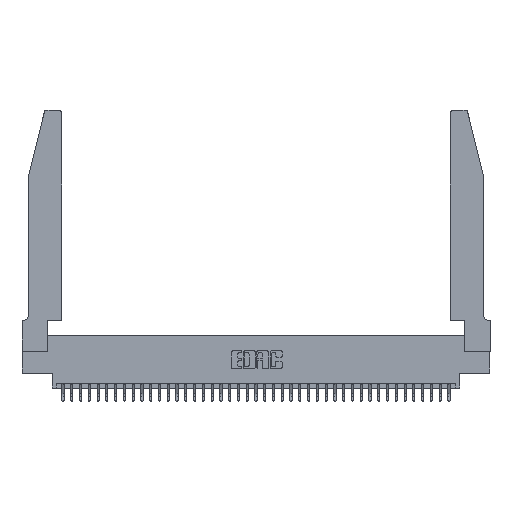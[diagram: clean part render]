
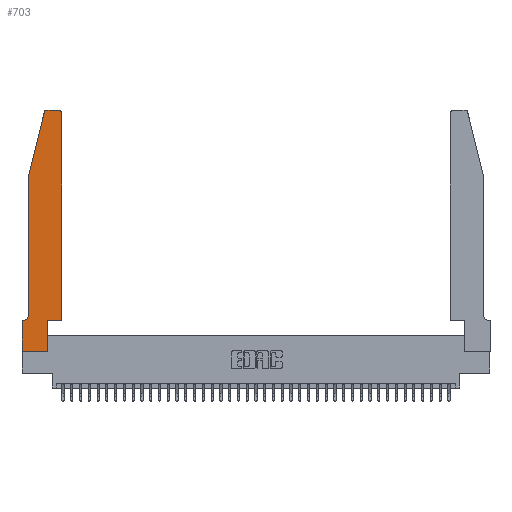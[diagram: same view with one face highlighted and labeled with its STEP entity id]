
A CAD part, top view. The second image highlights one B-rep face of the part: STEP entity #703.
In plain terms, the highlighted planar face has unit normal (0, 0, 1).
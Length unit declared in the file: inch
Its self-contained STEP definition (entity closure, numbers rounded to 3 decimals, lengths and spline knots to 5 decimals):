
#439 = LINE ( 'NONE', #4585, #27125 ) ;
#703 = ADVANCED_FACE ( 'NONE', ( #33845 ), #27674, .T. ) ;
#1113 = CARTESIAN_POINT ( 'NONE',  ( 0.2865, 0.35, 0.37 ) ) ;
#1779 = VECTOR ( 'NONE', #30031, 39.37008 ) ;
#1824 = AXIS2_PLACEMENT_3D ( 'NONE', #19420, #34696, #36988 ) ;
#2043 = CARTESIAN_POINT ( 'NONE',  ( 0., 0., 0.37 ) ) ;
#2507 = VERTEX_POINT ( 'NONE', #12022 ) ;
#2539 = VECTOR ( 'NONE', #35482, 39.37008 ) ;
#2873 = DIRECTION ( 'NONE',  ( -1., 0., 0. ) ) ;
#3063 = CARTESIAN_POINT ( 'NONE',  ( 0., 0., 0.37 ) ) ;
#3504 = VECTOR ( 'NONE', #10928, 39.37008 ) ;
#3772 = CARTESIAN_POINT ( 'NONE',  ( 0.0755, 0.35, 0.37 ) ) ;
#3827 = VERTEX_POINT ( 'NONE', #1113 ) ;
#4221 = CARTESIAN_POINT ( 'NONE',  ( 0.2865, 0., 0.37 ) ) ;
#4585 = CARTESIAN_POINT ( 'NONE',  ( 0.2605, 2.75, 0.37 ) ) ;
#4598 = EDGE_CURVE ( 'NONE', #10620, #25498, #7952, .T. ) ;
#5630 = LINE ( 'NONE', #7406, #1779 ) ;
#5864 = LINE ( 'NONE', #13849, #2539 ) ;
#6612 = EDGE_CURVE ( 'NONE', #27675, #13620, #20868, .T. ) ;
#7406 = CARTESIAN_POINT ( 'NONE',  ( 0.2865, 0.35, 0.37 ) ) ;
#7463 = EDGE_CURVE ( 'NONE', #13620, #33667, #439, .T. ) ;
#7952 = LINE ( 'NONE', #3772, #31646 ) ;
#8030 = ORIENTED_EDGE ( 'NONE', *, *, #7463, .T. ) ;
#8069 = LINE ( 'NONE', #9423, #23588 ) ;
#8191 = ORIENTED_EDGE ( 'NONE', *, *, #35374, .T. ) ;
#8224 = DIRECTION ( 'NONE',  ( 1., 0., 0. ) ) ;
#8551 = CIRCLE ( 'NONE', #23037, 0.07 ) ;
#8577 = ORIENTED_EDGE ( 'NONE', *, *, #36897, .T. ) ;
#8614 = DIRECTION ( 'NONE',  ( -1., 0., 0. ) ) ;
#8809 = CIRCLE ( 'NONE', #15777, 0.03 ) ;
#8848 = CARTESIAN_POINT ( 'NONE',  ( 0., 0.35, 0.37 ) ) ;
#9047 = ORIENTED_EDGE ( 'NONE', *, *, #6612, .T. ) ;
#9202 = ORIENTED_EDGE ( 'NONE', *, *, #4598, .T. ) ;
#9310 = EDGE_CURVE ( 'NONE', #33667, #2507, #8809, .T. ) ;
#9423 = CARTESIAN_POINT ( 'NONE',  ( 0.4505, 0.35, 0.37 ) ) ;
#10086 = ORIENTED_EDGE ( 'NONE', *, *, #12210, .T. ) ;
#10620 = VERTEX_POINT ( 'NONE', #23276 ) ;
#10928 = DIRECTION ( 'NONE',  ( 0., -1., 0. ) ) ;
#12022 = CARTESIAN_POINT ( 'NONE',  ( 0.25487, 2.72718, 0.37 ) ) ;
#12210 = EDGE_CURVE ( 'NONE', #12753, #39951, #36216, .T. ) ;
#12753 = VERTEX_POINT ( 'NONE', #2043 ) ;
#12763 = VERTEX_POINT ( 'NONE', #23956 ) ;
#13212 = EDGE_CURVE ( 'NONE', #39951, #3827, #5630, .T. ) ;
#13620 = VERTEX_POINT ( 'NONE', #39892 ) ;
#13668 = LINE ( 'NONE', #14161, #3504 ) ;
#13849 = CARTESIAN_POINT ( 'NONE',  ( 0.4505, 0.35, 0.37 ) ) ;
#14161 = CARTESIAN_POINT ( 'NONE',  ( 0.0755, 2., 0.37 ) ) ;
#15309 = DIRECTION ( 'NONE',  ( 0., 0., 1. ) ) ;
#15393 = DIRECTION ( 'NONE',  ( 0., 0., -1. ) ) ;
#15606 = ORIENTED_EDGE ( 'NONE', *, *, #9310, .T. ) ;
#15735 = DIRECTION ( 'NONE',  ( 0., 1., 0. ) ) ;
#15777 = AXIS2_PLACEMENT_3D ( 'NONE', #32325, #39075, #8224 ) ;
#16845 = EDGE_LOOP ( 'NONE', ( #8030, #15606, #8191, #22342, #34291, #9202, #8577, #10086, #24182, #27075, #36309, #9047 ) ) ;
#17397 = CARTESIAN_POINT ( 'NONE',  ( 0.0755, 2., 0.37 ) ) ;
#17480 = CARTESIAN_POINT ( 'NONE',  ( 0.0755, 2., 0.37 ) ) ;
#17711 = EDGE_CURVE ( 'NONE', #12763, #27675, #8069, .T. ) ;
#18636 = VECTOR ( 'NONE', #29467, 39.37008 ) ;
#19420 = CARTESIAN_POINT ( 'NONE',  ( 0.4205, 2.72, 0.37 ) ) ;
#19781 = AXIS2_PLACEMENT_3D ( 'NONE', #8848, #15309, #21330 ) ;
#20263 = CARTESIAN_POINT ( 'NONE',  ( 0., 0.35, 0.37 ) ) ;
#20697 = VERTEX_POINT ( 'NONE', #17480 ) ;
#20868 = CIRCLE ( 'NONE', #1824, 0.03 ) ;
#21330 = DIRECTION ( 'NONE',  ( 1., 0., 0. ) ) ;
#21413 = CARTESIAN_POINT ( 'NONE',  ( 0.0055, 0.42, 0.37 ) ) ;
#21728 = VECTOR ( 'NONE', #37864, 39.37008 ) ;
#22342 = ORIENTED_EDGE ( 'NONE', *, *, #22643, .T. ) ;
#22543 = LINE ( 'NONE', #17397, #18636 ) ;
#22643 = EDGE_CURVE ( 'NONE', #20697, #29456, #13668, .T. ) ;
#22699 = CARTESIAN_POINT ( 'NONE',  ( 0.0755, 0.42, 0.37 ) ) ;
#23037 = AXIS2_PLACEMENT_3D ( 'NONE', #21413, #15393, #2873 ) ;
#23184 = CARTESIAN_POINT ( 'NONE',  ( 0.284, 2.75, 0.37 ) ) ;
#23268 = EDGE_CURVE ( 'NONE', #3827, #12763, #5864, .T. ) ;
#23276 = CARTESIAN_POINT ( 'NONE',  ( 0.0055, 0.35, 0.37 ) ) ;
#23588 = VECTOR ( 'NONE', #15735, 39.37008 ) ;
#23956 = CARTESIAN_POINT ( 'NONE',  ( 0.4505, 0.35, 0.37 ) ) ;
#24182 = ORIENTED_EDGE ( 'NONE', *, *, #13212, .T. ) ;
#25498 = VERTEX_POINT ( 'NONE', #20263 ) ;
#27075 = ORIENTED_EDGE ( 'NONE', *, *, #23268, .T. ) ;
#27125 = VECTOR ( 'NONE', #8614, 39.37008 ) ;
#27674 = PLANE ( 'NONE',  #19781 ) ;
#27675 = VERTEX_POINT ( 'NONE', #34140 ) ;
#27693 = DIRECTION ( 'NONE',  ( 0., -1., 0. ) ) ;
#28401 = DIRECTION ( 'NONE',  ( -1., 0., 0. ) ) ;
#28715 = VECTOR ( 'NONE', #27693, 39.37008 ) ;
#29456 = VERTEX_POINT ( 'NONE', #22699 ) ;
#29467 = DIRECTION ( 'NONE',  ( -0.239, -0.971, 0. ) ) ;
#30031 = DIRECTION ( 'NONE',  ( 0., 1., 0. ) ) ;
#31646 = VECTOR ( 'NONE', #28401, 39.37008 ) ;
#32325 = CARTESIAN_POINT ( 'NONE',  ( 0.284, 2.72, 0.37 ) ) ;
#33667 = VERTEX_POINT ( 'NONE', #23184 ) ;
#33845 = FACE_OUTER_BOUND ( 'NONE', #16845, .T. ) ;
#34140 = CARTESIAN_POINT ( 'NONE',  ( 0.4505, 2.72, 0.37 ) ) ;
#34291 = ORIENTED_EDGE ( 'NONE', *, *, #34823, .T. ) ;
#34696 = DIRECTION ( 'NONE',  ( 0., 0., 1. ) ) ;
#34823 = EDGE_CURVE ( 'NONE', #29456, #10620, #8551, .T. ) ;
#35374 = EDGE_CURVE ( 'NONE', #2507, #20697, #22543, .T. ) ;
#35482 = DIRECTION ( 'NONE',  ( 1., 0., 0. ) ) ;
#36216 = LINE ( 'NONE', #37205, #21728 ) ;
#36309 = ORIENTED_EDGE ( 'NONE', *, *, #17711, .T. ) ;
#36897 = EDGE_CURVE ( 'NONE', #25498, #12753, #36940, .T. ) ;
#36940 = LINE ( 'NONE', #3063, #28715 ) ;
#36988 = DIRECTION ( 'NONE',  ( 1., 0., 0. ) ) ;
#37205 = CARTESIAN_POINT ( 'NONE',  ( 0., 0., 0.37 ) ) ;
#37864 = DIRECTION ( 'NONE',  ( 1., 0., 0. ) ) ;
#39075 = DIRECTION ( 'NONE',  ( 0., 0., 1. ) ) ;
#39892 = CARTESIAN_POINT ( 'NONE',  ( 0.4205, 2.75, 0.37 ) ) ;
#39951 = VERTEX_POINT ( 'NONE', #4221 ) ;
